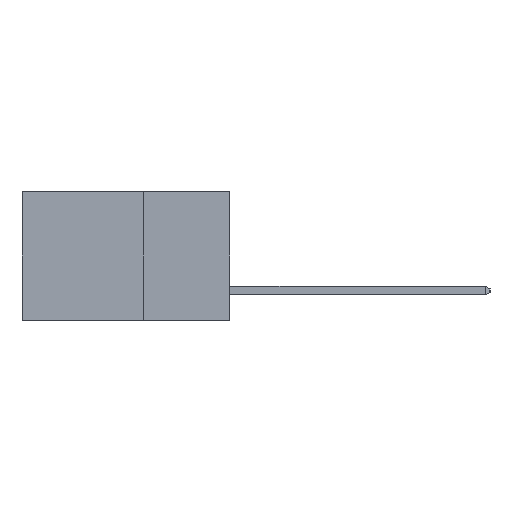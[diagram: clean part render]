
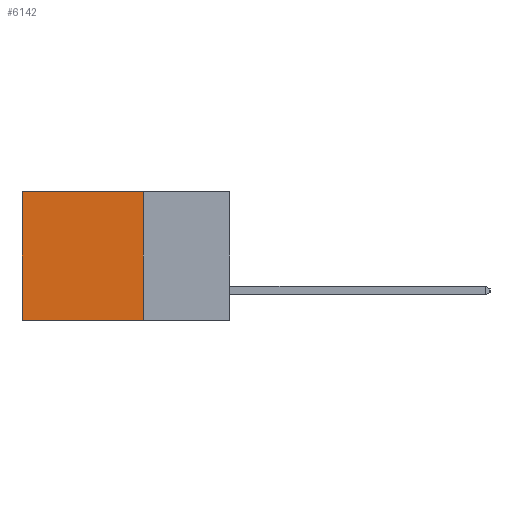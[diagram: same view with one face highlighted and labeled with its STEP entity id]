
A CAD part, left-side view. The second image highlights one B-rep face of the part: STEP entity #6142.
In plain terms, the highlighted planar face has unit normal (-1, 0, 0).
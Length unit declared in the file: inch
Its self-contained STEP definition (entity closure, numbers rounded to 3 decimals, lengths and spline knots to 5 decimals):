
#737 = EDGE_LOOP ( 'NONE', ( #13467, #9007, #16469, #16265 ) ) ;
#757 = LINE ( 'NONE', #19178, #18252 ) ;
#854 = DIRECTION ( 'NONE',  ( 0., 0., -1. ) ) ;
#975 = DIRECTION ( 'NONE',  ( 0., 1., 0. ) ) ;
#1136 = AXIS2_PLACEMENT_3D ( 'NONE', #17601, #17456, #3597 ) ;
#1598 = EDGE_CURVE ( 'NONE', #20323, #21245, #757, .T. ) ;
#2034 = PLANE ( 'NONE',  #1136 ) ;
#3597 = DIRECTION ( 'NONE',  ( 0., 0., -1. ) ) ;
#4632 = CARTESIAN_POINT ( 'NONE',  ( 0.298, 0.6, 0. ) ) ;
#4640 = LINE ( 'NONE', #11288, #17516 ) ;
#5355 = EDGE_CURVE ( 'NONE', #20310, #21245, #19507, .T. ) ;
#6142 = ADVANCED_FACE ( 'NONE', ( #13853 ), #2034, .F. ) ;
#8724 = CARTESIAN_POINT ( 'NONE',  ( 0.298, 0.6, -0.37 ) ) ;
#9007 = ORIENTED_EDGE ( 'NONE', *, *, #1598, .F. ) ;
#9705 = CARTESIAN_POINT ( 'NONE',  ( 0.298, 0.25, -0.37 ) ) ;
#10758 = CARTESIAN_POINT ( 'NONE',  ( 0.298, 0.25, 0. ) ) ;
#11288 = CARTESIAN_POINT ( 'NONE',  ( 0.298, 0.25, 0. ) ) ;
#12114 = EDGE_CURVE ( 'NONE', #16916, #20323, #4640, .T. ) ;
#12438 = LINE ( 'NONE', #16229, #16311 ) ;
#13467 = ORIENTED_EDGE ( 'NONE', *, *, #5355, .T. ) ;
#13853 = FACE_OUTER_BOUND ( 'NONE', #737, .T. ) ;
#14652 = CARTESIAN_POINT ( 'NONE',  ( 0.298, 0.6, 0. ) ) ;
#14713 = DIRECTION ( 'NONE',  ( 0., 0., -1. ) ) ;
#15142 = VECTOR ( 'NONE', #854, 39.37008 ) ;
#16229 = CARTESIAN_POINT ( 'NONE',  ( 0.298, 0.25, 0. ) ) ;
#16265 = ORIENTED_EDGE ( 'NONE', *, *, #20915, .T. ) ;
#16311 = VECTOR ( 'NONE', #975, 39.37008 ) ;
#16469 = ORIENTED_EDGE ( 'NONE', *, *, #12114, .F. ) ;
#16916 = VERTEX_POINT ( 'NONE', #10758 ) ;
#17309 = DIRECTION ( 'NONE',  ( 0., 1., 0. ) ) ;
#17456 = DIRECTION ( 'NONE',  ( 1., 0., 0. ) ) ;
#17516 = VECTOR ( 'NONE', #14713, 39.37008 ) ;
#17601 = CARTESIAN_POINT ( 'NONE',  ( 0.298, 0.25, 0. ) ) ;
#18252 = VECTOR ( 'NONE', #17309, 39.37008 ) ;
#19178 = CARTESIAN_POINT ( 'NONE',  ( 0.298, 0.25, -0.37 ) ) ;
#19507 = LINE ( 'NONE', #14652, #15142 ) ;
#20310 = VERTEX_POINT ( 'NONE', #4632 ) ;
#20323 = VERTEX_POINT ( 'NONE', #9705 ) ;
#20915 = EDGE_CURVE ( 'NONE', #16916, #20310, #12438, .T. ) ;
#21245 = VERTEX_POINT ( 'NONE', #8724 ) ;
